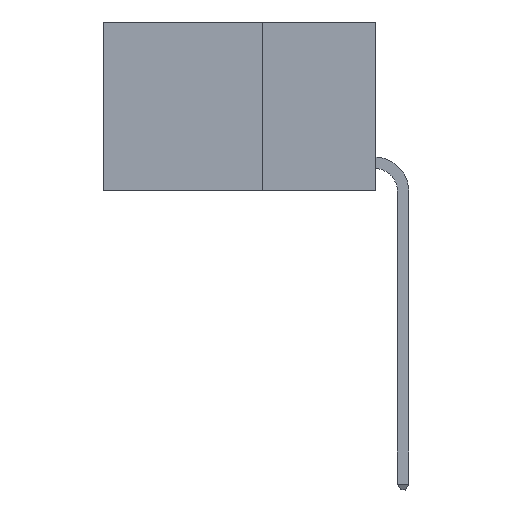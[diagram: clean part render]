
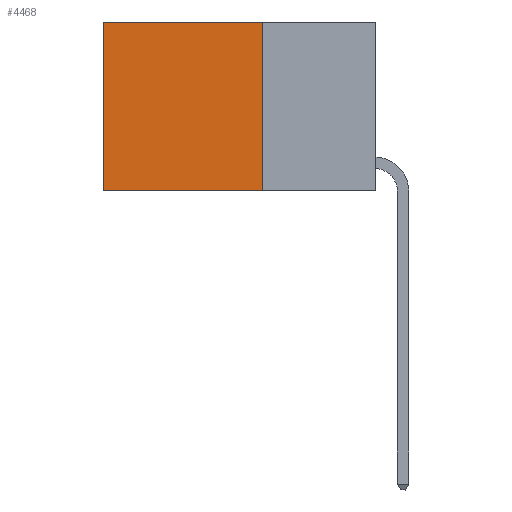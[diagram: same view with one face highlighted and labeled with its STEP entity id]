
A CAD part, left-side view. The second image highlights one B-rep face of the part: STEP entity #4468.
In plain terms, the highlighted planar face has unit normal (-1, 0, 0).
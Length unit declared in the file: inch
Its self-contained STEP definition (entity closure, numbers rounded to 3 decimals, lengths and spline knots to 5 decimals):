
#208 = EDGE_LOOP ( 'NONE', ( #8757, #3961, #1767, #11524 ) ) ;
#918 = DIRECTION ( 'NONE',  ( 1., 0., 0. ) ) ;
#919 = LINE ( 'NONE', #8881, #3375 ) ;
#1755 = AXIS2_PLACEMENT_3D ( 'NONE', #1924, #918, #8355 ) ;
#1767 = ORIENTED_EDGE ( 'NONE', *, *, #4401, .F. ) ;
#1924 = CARTESIAN_POINT ( 'NONE',  ( 0.2625, 0.25, 0. ) ) ;
#1950 = LINE ( 'NONE', #13266, #12718 ) ;
#2025 = VECTOR ( 'NONE', #5878, 39.37008 ) ;
#3375 = VECTOR ( 'NONE', #3577, 39.37008 ) ;
#3577 = DIRECTION ( 'NONE',  ( 0., 0., -1. ) ) ;
#3759 = FACE_OUTER_BOUND ( 'NONE', #208, .T. ) ;
#3961 = ORIENTED_EDGE ( 'NONE', *, *, #8466, .F. ) ;
#3972 = DIRECTION ( 'NONE',  ( 0., 0., -1. ) ) ;
#4076 = PLANE ( 'NONE',  #1755 ) ;
#4401 = EDGE_CURVE ( 'NONE', #10124, #4692, #1950, .T. ) ;
#4468 = ADVANCED_FACE ( 'NONE', ( #3759 ), #4076, .F. ) ;
#4692 = VERTEX_POINT ( 'NONE', #12729 ) ;
#5878 = DIRECTION ( 'NONE',  ( 0., 1., 0. ) ) ;
#7017 = LINE ( 'NONE', #11079, #2025 ) ;
#7970 = EDGE_CURVE ( 'NONE', #10124, #13454, #11118, .T. ) ;
#8079 = VERTEX_POINT ( 'NONE', #13460 ) ;
#8268 = CARTESIAN_POINT ( 'NONE',  ( 0.2625, 0.25, 0. ) ) ;
#8355 = DIRECTION ( 'NONE',  ( 0., 0., -1. ) ) ;
#8466 = EDGE_CURVE ( 'NONE', #4692, #8079, #7017, .T. ) ;
#8718 = CARTESIAN_POINT ( 'NONE',  ( 0.2625, 0.6, 0. ) ) ;
#8757 = ORIENTED_EDGE ( 'NONE', *, *, #12585, .T. ) ;
#8881 = CARTESIAN_POINT ( 'NONE',  ( 0.2625, 0.6, 0. ) ) ;
#10124 = VERTEX_POINT ( 'NONE', #11086 ) ;
#10502 = VECTOR ( 'NONE', #13324, 39.37008 ) ;
#11079 = CARTESIAN_POINT ( 'NONE',  ( 0.2625, 0.25, -0.37 ) ) ;
#11086 = CARTESIAN_POINT ( 'NONE',  ( 0.2625, 0.25, 0. ) ) ;
#11118 = LINE ( 'NONE', #8268, #10502 ) ;
#11524 = ORIENTED_EDGE ( 'NONE', *, *, #7970, .T. ) ;
#12585 = EDGE_CURVE ( 'NONE', #13454, #8079, #919, .T. ) ;
#12718 = VECTOR ( 'NONE', #3972, 39.37008 ) ;
#12729 = CARTESIAN_POINT ( 'NONE',  ( 0.2625, 0.25, -0.37 ) ) ;
#13266 = CARTESIAN_POINT ( 'NONE',  ( 0.2625, 0.25, 0. ) ) ;
#13324 = DIRECTION ( 'NONE',  ( 0., 1., 0. ) ) ;
#13454 = VERTEX_POINT ( 'NONE', #8718 ) ;
#13460 = CARTESIAN_POINT ( 'NONE',  ( 0.2625, 0.6, -0.37 ) ) ;
